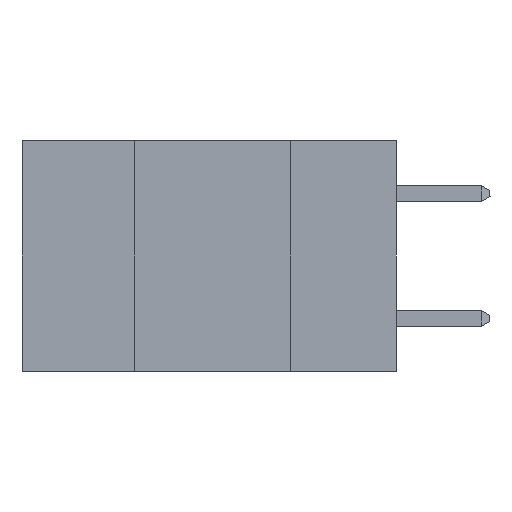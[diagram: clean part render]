
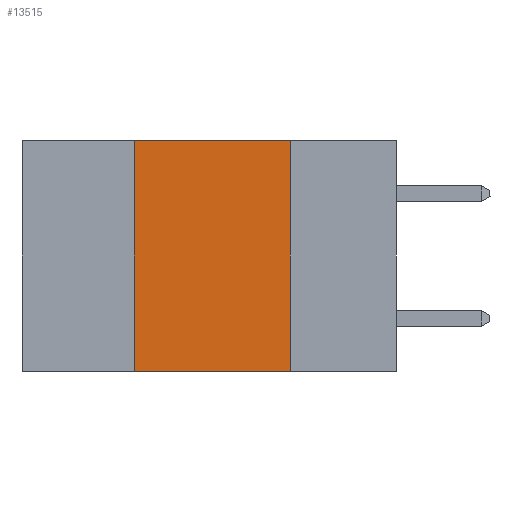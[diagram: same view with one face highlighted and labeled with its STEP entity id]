
A CAD part, left-side view. The second image highlights one B-rep face of the part: STEP entity #13515.
In plain terms, the highlighted planar face has unit normal (-1, 0, 0).
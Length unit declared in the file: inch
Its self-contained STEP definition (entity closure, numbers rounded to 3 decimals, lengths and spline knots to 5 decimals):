
#1331 = LINE ( 'NONE', #5727, #2205 ) ;
#2129 = FACE_OUTER_BOUND ( 'NONE', #12675, .T. ) ;
#2205 = VECTOR ( 'NONE', #7176, 39.37008 ) ;
#3122 = CARTESIAN_POINT ( 'NONE',  ( 0., 0.42, 0. ) ) ;
#3635 = LINE ( 'NONE', #6412, #11479 ) ;
#3864 = LINE ( 'NONE', #17711, #5603 ) ;
#4107 = CARTESIAN_POINT ( 'NONE',  ( 0., 0.17, 0. ) ) ;
#4837 = EDGE_CURVE ( 'NONE', #8652, #16377, #1331, .T. ) ;
#5217 = ORIENTED_EDGE ( 'NONE', *, *, #12786, .T. ) ;
#5603 = VECTOR ( 'NONE', #12333, 39.37008 ) ;
#5727 = CARTESIAN_POINT ( 'NONE',  ( 0., 0.6, 0. ) ) ;
#6412 = CARTESIAN_POINT ( 'NONE',  ( 0., 0.6, -0.37 ) ) ;
#6805 = VERTEX_POINT ( 'NONE', #14957 ) ;
#6857 = LINE ( 'NONE', #16076, #16837 ) ;
#7042 = DIRECTION ( 'NONE',  ( 1., 0., 0. ) ) ;
#7176 = DIRECTION ( 'NONE',  ( 0., -1., 0. ) ) ;
#7793 = DIRECTION ( 'NONE',  ( 0., 0., 1. ) ) ;
#8116 = ORIENTED_EDGE ( 'NONE', *, *, #12389, .F. ) ;
#8232 = CARTESIAN_POINT ( 'NONE',  ( 0., 0.6, 0. ) ) ;
#8363 = PLANE ( 'NONE',  #15363 ) ;
#8652 = VERTEX_POINT ( 'NONE', #3122 ) ;
#9347 = DIRECTION ( 'NONE',  ( 0., -1., 0. ) ) ;
#9661 = DIRECTION ( 'NONE',  ( 0., 0., -1. ) ) ;
#10868 = ORIENTED_EDGE ( 'NONE', *, *, #12864, .F. ) ;
#11479 = VECTOR ( 'NONE', #9347, 39.37008 ) ;
#11997 = VERTEX_POINT ( 'NONE', #15896 ) ;
#12333 = DIRECTION ( 'NONE',  ( 0., 0., -1. ) ) ;
#12389 = EDGE_CURVE ( 'NONE', #16377, #6805, #3864, .T. ) ;
#12675 = EDGE_LOOP ( 'NONE', ( #8116, #15165, #10868, #5217 ) ) ;
#12786 = EDGE_CURVE ( 'NONE', #11997, #6805, #3635, .T. ) ;
#12864 = EDGE_CURVE ( 'NONE', #11997, #8652, #6857, .T. ) ;
#13515 = ADVANCED_FACE ( 'NONE', ( #2129 ), #8363, .F. ) ;
#14957 = CARTESIAN_POINT ( 'NONE',  ( 0., 0.17, -0.37 ) ) ;
#15165 = ORIENTED_EDGE ( 'NONE', *, *, #4837, .F. ) ;
#15363 = AXIS2_PLACEMENT_3D ( 'NONE', #8232, #7042, #9661 ) ;
#15896 = CARTESIAN_POINT ( 'NONE',  ( 0., 0.42, -0.37 ) ) ;
#16076 = CARTESIAN_POINT ( 'NONE',  ( 0., 0.42, 0. ) ) ;
#16377 = VERTEX_POINT ( 'NONE', #4107 ) ;
#16837 = VECTOR ( 'NONE', #7793, 39.37008 ) ;
#17711 = CARTESIAN_POINT ( 'NONE',  ( 0., 0.17, 0. ) ) ;
